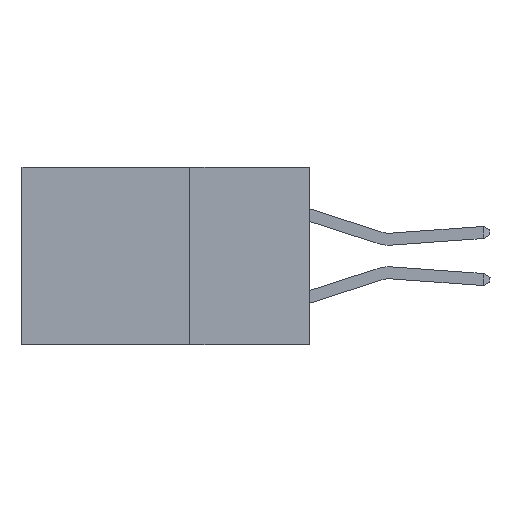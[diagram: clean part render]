
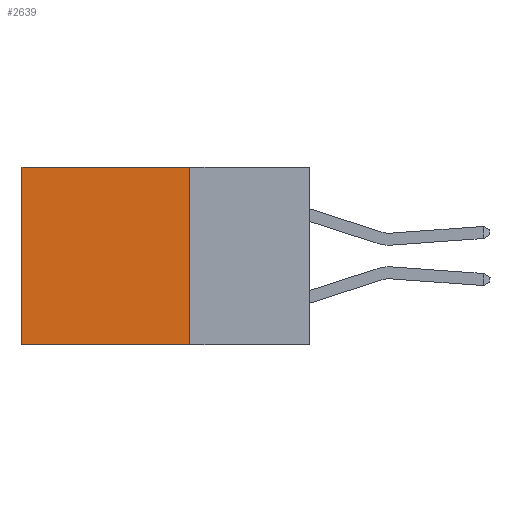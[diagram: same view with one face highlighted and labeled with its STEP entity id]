
A CAD part, left-side view. The second image highlights one B-rep face of the part: STEP entity #2639.
In plain terms, the highlighted planar face has unit normal (-1, 0, 0).
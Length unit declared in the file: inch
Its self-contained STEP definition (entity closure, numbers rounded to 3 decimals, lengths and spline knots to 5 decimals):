
#291 = LINE ( 'NONE', #11437, #13250 ) ;
#475 = VERTEX_POINT ( 'NONE', #15737 ) ;
#836 = LINE ( 'NONE', #6162, #8939 ) ;
#1137 = EDGE_CURVE ( 'NONE', #475, #6309, #13770, .T. ) ;
#1519 = DIRECTION ( 'NONE',  ( 1., 0., 0. ) ) ;
#2400 = LINE ( 'NONE', #16760, #19074 ) ;
#2639 = ADVANCED_FACE ( 'NONE', ( #5876 ), #5799, .F. ) ;
#4285 = VERTEX_POINT ( 'NONE', #16478 ) ;
#4825 = CARTESIAN_POINT ( 'NONE',  ( 0.298, 0.25, -0.37 ) ) ;
#4830 = DIRECTION ( 'NONE',  ( 0., 1., 0. ) ) ;
#4934 = VERTEX_POINT ( 'NONE', #8530 ) ;
#5535 = ORIENTED_EDGE ( 'NONE', *, *, #8886, .T. ) ;
#5799 = PLANE ( 'NONE',  #15409 ) ;
#5876 = FACE_OUTER_BOUND ( 'NONE', #20432, .T. ) ;
#6162 = CARTESIAN_POINT ( 'NONE',  ( 0.298, 0.6, 0. ) ) ;
#6309 = VERTEX_POINT ( 'NONE', #12437 ) ;
#6519 = CARTESIAN_POINT ( 'NONE',  ( 0.298, 0.25, 0. ) ) ;
#6755 = EDGE_CURVE ( 'NONE', #4285, #4934, #2400, .T. ) ;
#8053 = DIRECTION ( 'NONE',  ( 0., 0., -1. ) ) ;
#8202 = DIRECTION ( 'NONE',  ( 0., 0., -1. ) ) ;
#8322 = ORIENTED_EDGE ( 'NONE', *, *, #15593, .F. ) ;
#8530 = CARTESIAN_POINT ( 'NONE',  ( 0.298, 0.6, 0. ) ) ;
#8557 = ORIENTED_EDGE ( 'NONE', *, *, #1137, .F. ) ;
#8886 = EDGE_CURVE ( 'NONE', #4934, #6309, #836, .T. ) ;
#8939 = VECTOR ( 'NONE', #17457, 39.37008 ) ;
#10299 = DIRECTION ( 'NONE',  ( 0., 1., 0. ) ) ;
#11437 = CARTESIAN_POINT ( 'NONE',  ( 0.298, 0.25, 0. ) ) ;
#12437 = CARTESIAN_POINT ( 'NONE',  ( 0.298, 0.6, -0.37 ) ) ;
#13250 = VECTOR ( 'NONE', #8202, 39.37008 ) ;
#13424 = ORIENTED_EDGE ( 'NONE', *, *, #6755, .T. ) ;
#13770 = LINE ( 'NONE', #4825, #17558 ) ;
#15409 = AXIS2_PLACEMENT_3D ( 'NONE', #6519, #1519, #8053 ) ;
#15593 = EDGE_CURVE ( 'NONE', #4285, #475, #291, .T. ) ;
#15737 = CARTESIAN_POINT ( 'NONE',  ( 0.298, 0.25, -0.37 ) ) ;
#16478 = CARTESIAN_POINT ( 'NONE',  ( 0.298, 0.25, 0. ) ) ;
#16760 = CARTESIAN_POINT ( 'NONE',  ( 0.298, 0.25, 0. ) ) ;
#17457 = DIRECTION ( 'NONE',  ( 0., 0., -1. ) ) ;
#17558 = VECTOR ( 'NONE', #4830, 39.37008 ) ;
#19074 = VECTOR ( 'NONE', #10299, 39.37008 ) ;
#20432 = EDGE_LOOP ( 'NONE', ( #5535, #8557, #8322, #13424 ) ) ;
